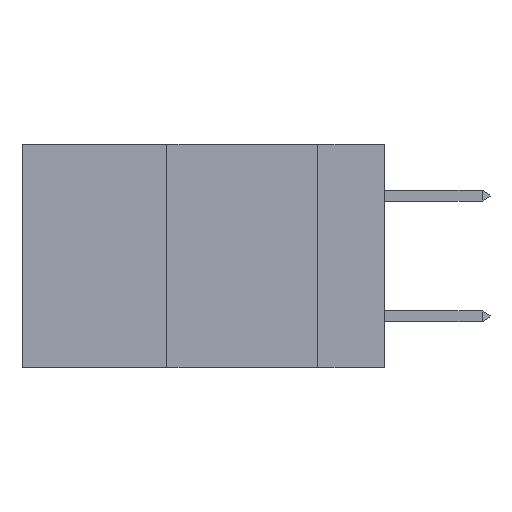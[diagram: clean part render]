
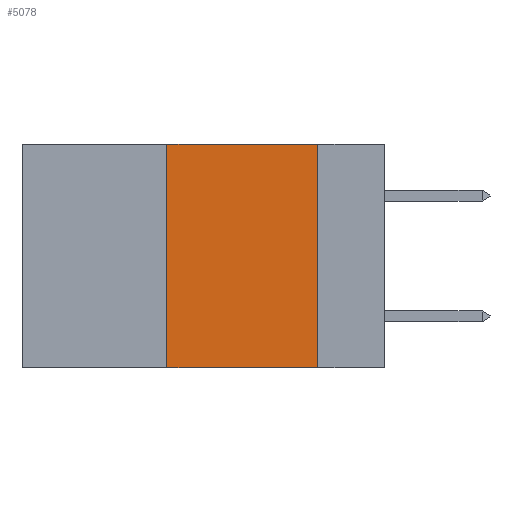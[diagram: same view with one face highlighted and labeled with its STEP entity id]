
A CAD part, left-side view. The second image highlights one B-rep face of the part: STEP entity #5078.
In plain terms, the highlighted planar face has unit normal (-1, 0, 0).
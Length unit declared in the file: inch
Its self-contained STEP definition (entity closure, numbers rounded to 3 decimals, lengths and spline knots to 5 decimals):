
#2017 = VECTOR ( 'NONE', #5125, 39.37008 ) ;
#2287 = ORIENTED_EDGE ( 'NONE', *, *, #8896, .F. ) ;
#2352 = DIRECTION ( 'NONE',  ( 0., -1., 0. ) ) ;
#2376 = PLANE ( 'NONE',  #20693 ) ;
#2390 = DIRECTION ( 'NONE',  ( 0., 0., -1. ) ) ;
#2868 = VERTEX_POINT ( 'NONE', #5118 ) ;
#3461 = VERTEX_POINT ( 'NONE', #7489 ) ;
#3540 = CARTESIAN_POINT ( 'NONE',  ( 0., 0.11, -0.37 ) ) ;
#3833 = DIRECTION ( 'NONE',  ( 1., 0., 0. ) ) ;
#4391 = LINE ( 'NONE', #5728, #10401 ) ;
#4653 = VECTOR ( 'NONE', #5775, 39.37008 ) ;
#4964 = FACE_OUTER_BOUND ( 'NONE', #16767, .T. ) ;
#5078 = ADVANCED_FACE ( 'NONE', ( #4964 ), #2376, .F. ) ;
#5118 = CARTESIAN_POINT ( 'NONE',  ( 0., 0.36, 0. ) ) ;
#5125 = DIRECTION ( 'NONE',  ( 0., -1., 0. ) ) ;
#5728 = CARTESIAN_POINT ( 'NONE',  ( 0., 0.11, 0. ) ) ;
#5775 = DIRECTION ( 'NONE',  ( 0., 0., 1. ) ) ;
#7011 = EDGE_CURVE ( 'NONE', #3461, #16778, #8900, .T. ) ;
#7100 = CARTESIAN_POINT ( 'NONE',  ( 0., 0.36, 0. ) ) ;
#7489 = CARTESIAN_POINT ( 'NONE',  ( 0., 0.36, -0.37 ) ) ;
#8896 = EDGE_CURVE ( 'NONE', #3461, #2868, #12531, .T. ) ;
#8900 = LINE ( 'NONE', #21021, #16660 ) ;
#9143 = DIRECTION ( 'NONE',  ( 0., 0., -1. ) ) ;
#9788 = CARTESIAN_POINT ( 'NONE',  ( 0., 0.11, 0. ) ) ;
#10401 = VECTOR ( 'NONE', #2390, 39.37008 ) ;
#11654 = ORIENTED_EDGE ( 'NONE', *, *, #11756, .F. ) ;
#11756 = EDGE_CURVE ( 'NONE', #14449, #16778, #4391, .T. ) ;
#12531 = LINE ( 'NONE', #7100, #4653 ) ;
#13975 = ORIENTED_EDGE ( 'NONE', *, *, #7011, .T. ) ;
#14247 = CARTESIAN_POINT ( 'NONE',  ( 0., 0.6, 0. ) ) ;
#14449 = VERTEX_POINT ( 'NONE', #9788 ) ;
#14656 = ORIENTED_EDGE ( 'NONE', *, *, #17542, .F. ) ;
#16660 = VECTOR ( 'NONE', #2352, 39.37008 ) ;
#16767 = EDGE_LOOP ( 'NONE', ( #11654, #14656, #2287, #13975 ) ) ;
#16778 = VERTEX_POINT ( 'NONE', #3540 ) ;
#17542 = EDGE_CURVE ( 'NONE', #2868, #14449, #18882, .T. ) ;
#18882 = LINE ( 'NONE', #20323, #2017 ) ;
#20323 = CARTESIAN_POINT ( 'NONE',  ( 0., 0.6, 0. ) ) ;
#20693 = AXIS2_PLACEMENT_3D ( 'NONE', #14247, #3833, #9143 ) ;
#21021 = CARTESIAN_POINT ( 'NONE',  ( 0., 0.6, -0.37 ) ) ;
